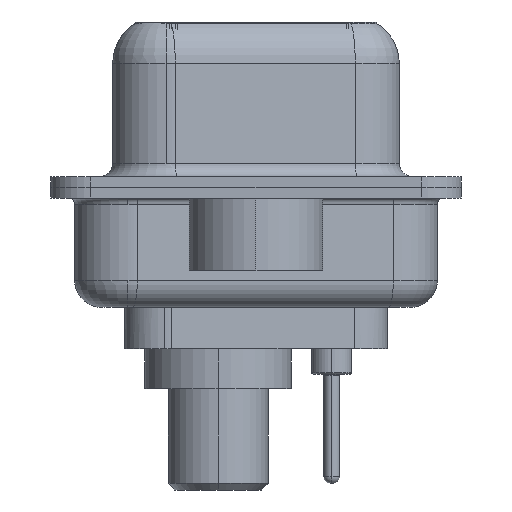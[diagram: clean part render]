
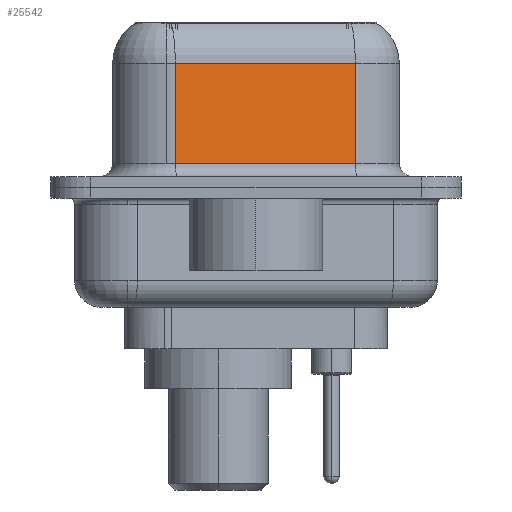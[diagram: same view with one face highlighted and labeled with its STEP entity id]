
A CAD part, left-side view. The second image highlights one B-rep face of the part: STEP entity #25542.
In plain terms, the highlighted planar face has unit normal (-0.985, -0.174, 0).
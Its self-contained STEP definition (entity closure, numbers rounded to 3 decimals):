
#740 = CARTESIAN_POINT ( 'NONE',  ( 4.43, 3.028, 6.4 ) ) ;
#2219 = EDGE_CURVE ( 'NONE', #19442, #4105, #24147, .T. ) ;
#4105 = VERTEX_POINT ( 'NONE', #5367 ) ;
#5367 = CARTESIAN_POINT ( 'NONE',  ( 5.621, -3.722, 0.9 ) ) ;
#7285 = DIRECTION ( 'NONE',  ( -0.174, 0.985, 0. ) ) ;
#8195 = VECTOR ( 'NONE', #30615, 1000. ) ;
#8290 = PLANE ( 'NONE',  #28318 ) ;
#12545 = VERTEX_POINT ( 'NONE', #33763 ) ;
#12564 = EDGE_CURVE ( 'NONE', #22384, #12545, #19841, .T. ) ;
#12750 = VECTOR ( 'NONE', #21765, 1000. ) ;
#15801 = VECTOR ( 'NONE', #7285, 1000. ) ;
#16164 = CARTESIAN_POINT ( 'NONE',  ( 5.621, -3.722, 6.4 ) ) ;
#16992 = VECTOR ( 'NONE', #22218, 1000. ) ;
#17670 = LINE ( 'NONE', #740, #12750 ) ;
#18057 = ORIENTED_EDGE ( 'NONE', *, *, #2219, .T. ) ;
#19442 = VERTEX_POINT ( 'NONE', #23882 ) ;
#19841 = LINE ( 'NONE', #28605, #15801 ) ;
#20131 = CARTESIAN_POINT ( 'NONE',  ( 5.621, -3.722, 4.65 ) ) ;
#20588 = CARTESIAN_POINT ( 'NONE',  ( 5.621, -3.722, 0.9 ) ) ;
#21512 = LINE ( 'NONE', #27396, #16992 ) ;
#21765 = DIRECTION ( 'NONE',  ( 0., 0., -1. ) ) ;
#22218 = DIRECTION ( 'NONE',  ( 0., 0., -1. ) ) ;
#22384 = VERTEX_POINT ( 'NONE', #20131 ) ;
#22725 = ORIENTED_EDGE ( 'NONE', *, *, #25160, .F. ) ;
#23882 = CARTESIAN_POINT ( 'NONE',  ( 4.43, 3.028, 0.9 ) ) ;
#24147 = LINE ( 'NONE', #20588, #8195 ) ;
#25160 = EDGE_CURVE ( 'NONE', #22384, #4105, #21512, .T. ) ;
#25228 = FACE_OUTER_BOUND ( 'NONE', #28564, .T. ) ;
#25542 = ADVANCED_FACE ( 'NONE', ( #25228 ), #8290, .F. ) ;
#27349 = EDGE_CURVE ( 'NONE', #12545, #19442, #17670, .T. ) ;
#27396 = CARTESIAN_POINT ( 'NONE',  ( 5.621, -3.722, 6.4 ) ) ;
#28318 = AXIS2_PLACEMENT_3D ( 'NONE', #16164, #28923, #29160 ) ;
#28564 = EDGE_LOOP ( 'NONE', ( #22725, #31648, #29350, #18057 ) ) ;
#28605 = CARTESIAN_POINT ( 'NONE',  ( 5.621, -3.722, 4.65 ) ) ;
#28923 = DIRECTION ( 'NONE',  ( 0.985, 0.174, 0. ) ) ;
#29160 = DIRECTION ( 'NONE',  ( -0.174, 0.985, 0. ) ) ;
#29350 = ORIENTED_EDGE ( 'NONE', *, *, #27349, .T. ) ;
#30615 = DIRECTION ( 'NONE',  ( 0.174, -0.985, 0. ) ) ;
#31648 = ORIENTED_EDGE ( 'NONE', *, *, #12564, .T. ) ;
#33763 = CARTESIAN_POINT ( 'NONE',  ( 4.43, 3.028, 4.65 ) ) ;
